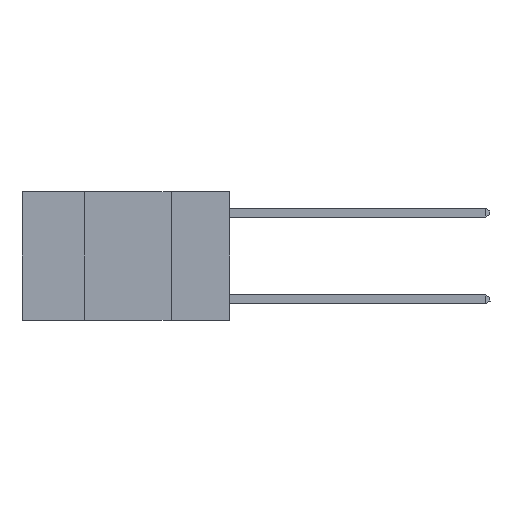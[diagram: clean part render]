
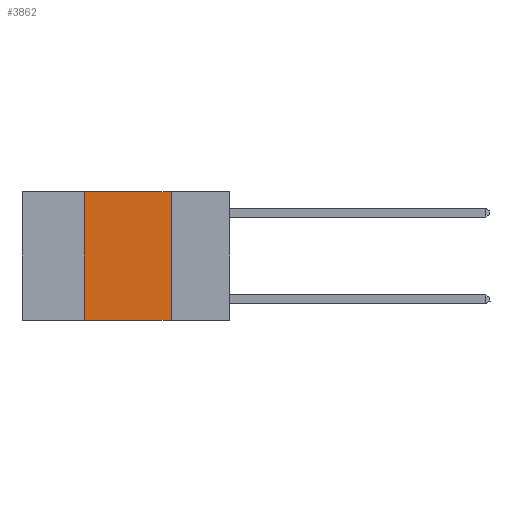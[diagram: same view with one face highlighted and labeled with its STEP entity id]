
A CAD part, left-side view. The second image highlights one B-rep face of the part: STEP entity #3862.
In plain terms, the highlighted planar face has unit normal (-1, 0, 0).
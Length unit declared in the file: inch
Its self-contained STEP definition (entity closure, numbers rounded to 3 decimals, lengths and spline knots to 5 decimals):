
#581 = EDGE_CURVE ( 'NONE', #4943, #5644, #9471, .T. ) ;
#901 = CARTESIAN_POINT ( 'NONE',  ( 0., 0.6, 0. ) ) ;
#1185 = VECTOR ( 'NONE', #6485, 39.37008 ) ;
#1487 = CARTESIAN_POINT ( 'NONE',  ( 0., 0.42, -0.37 ) ) ;
#2188 = CARTESIAN_POINT ( 'NONE',  ( 0., 0.17, -0.37 ) ) ;
#2274 = ORIENTED_EDGE ( 'NONE', *, *, #2407, .F. ) ;
#2407 = EDGE_CURVE ( 'NONE', #7541, #11892, #10432, .T. ) ;
#2607 = ORIENTED_EDGE ( 'NONE', *, *, #581, .F. ) ;
#2701 = CARTESIAN_POINT ( 'NONE',  ( 0., 0.17, 0. ) ) ;
#3300 = DIRECTION ( 'NONE',  ( 0., -1., 0. ) ) ;
#3339 = VECTOR ( 'NONE', #3300, 39.37008 ) ;
#3862 = ADVANCED_FACE ( 'NONE', ( #12352 ), #12129, .F. ) ;
#4162 = ORIENTED_EDGE ( 'NONE', *, *, #11943, .T. ) ;
#4632 = EDGE_CURVE ( 'NONE', #5644, #7541, #9459, .T. ) ;
#4938 = CARTESIAN_POINT ( 'NONE',  ( 0., 0.42, 0. ) ) ;
#4943 = VERTEX_POINT ( 'NONE', #1487 ) ;
#5072 = VECTOR ( 'NONE', #7452, 39.37008 ) ;
#5403 = CARTESIAN_POINT ( 'NONE',  ( 0., 0.6, 0. ) ) ;
#5644 = VERTEX_POINT ( 'NONE', #4938 ) ;
#6163 = LINE ( 'NONE', #8508, #3339 ) ;
#6485 = DIRECTION ( 'NONE',  ( 0., -1., 0. ) ) ;
#6977 = DIRECTION ( 'NONE',  ( 0., 0., 1. ) ) ;
#7115 = VECTOR ( 'NONE', #6977, 39.37008 ) ;
#7223 = DIRECTION ( 'NONE',  ( 0., 0., -1. ) ) ;
#7377 = CARTESIAN_POINT ( 'NONE',  ( 0., 0.17, 0. ) ) ;
#7452 = DIRECTION ( 'NONE',  ( 0., 0., -1. ) ) ;
#7541 = VERTEX_POINT ( 'NONE', #2701 ) ;
#7866 = ORIENTED_EDGE ( 'NONE', *, *, #4632, .F. ) ;
#8508 = CARTESIAN_POINT ( 'NONE',  ( 0., 0.6, -0.37 ) ) ;
#9330 = AXIS2_PLACEMENT_3D ( 'NONE', #901, #13056, #7223 ) ;
#9459 = LINE ( 'NONE', #5403, #1185 ) ;
#9471 = LINE ( 'NONE', #12583, #7115 ) ;
#10089 = EDGE_LOOP ( 'NONE', ( #2274, #7866, #2607, #4162 ) ) ;
#10432 = LINE ( 'NONE', #7377, #5072 ) ;
#11892 = VERTEX_POINT ( 'NONE', #2188 ) ;
#11943 = EDGE_CURVE ( 'NONE', #4943, #11892, #6163, .T. ) ;
#12129 = PLANE ( 'NONE',  #9330 ) ;
#12352 = FACE_OUTER_BOUND ( 'NONE', #10089, .T. ) ;
#12583 = CARTESIAN_POINT ( 'NONE',  ( 0., 0.42, 0. ) ) ;
#13056 = DIRECTION ( 'NONE',  ( 1., 0., 0. ) ) ;
